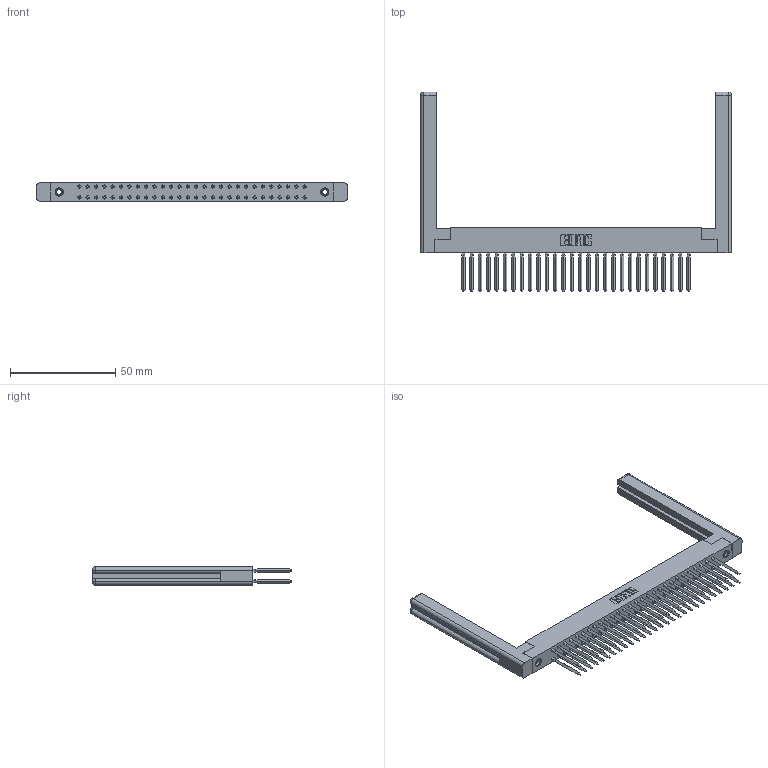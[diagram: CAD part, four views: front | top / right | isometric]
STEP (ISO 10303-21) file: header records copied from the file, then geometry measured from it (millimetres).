
FILE_DESCRIPTION (( 'STEP AP203' ), '1' );
FILE_NAME ('338-056-541-258.STEP', '2020-03-24T18:58:20', ( '' ), ( '' ), 'SwSTEP 2.0', 'SolidWorks 2016', '' );
FILE_SCHEMA (( 'CONFIG_CONTROL_DESIGN' ));
Length unit declared in the file: inch
Products named in the file (5): 345-250-001_345-250-001-102; 338-290-001_541; 338-056-541-258; 307-220-058; 338-210-001_338-210-028-004
Assembly tree (61 placements, depth 2):
  338-056-541-258
    338-210-001_338-210-028-004
    338-290-001_541  x56
    345-250-001_345-250-001-102  x2
    307-220-058  x2
Bounding box: 147.57 x 94.87 x 8.71 mm (x, y, z)
Volume: 18933 mm3; surface area: 26175.8 mm2
Topology: 61 solids, 61 shells, 3988 faces, 10685 edges, 6774 vertices
Faces by surface type: plane 2766, cylinder 974, bspline 224, cone 12, torus 12
Entity records: 58641 total; most frequent: CARTESIAN_POINT 11555, ORIENTED_EDGE 9722, DIRECTION 9156, EDGE_CURVE 4861, LINE 3634, VECTOR 3634, VERTEX_POINT 3154, AXIS2_PLACEMENT_3D 2761
